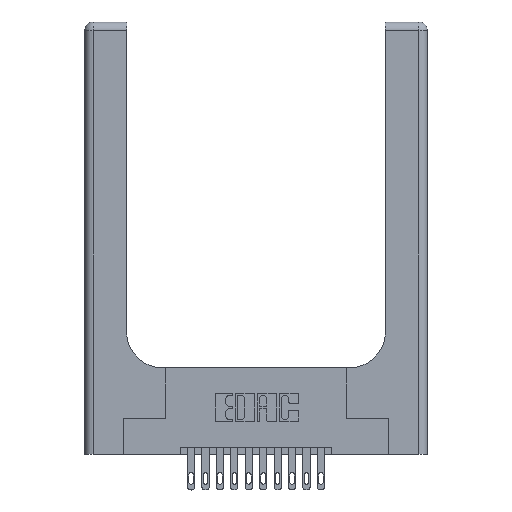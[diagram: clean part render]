
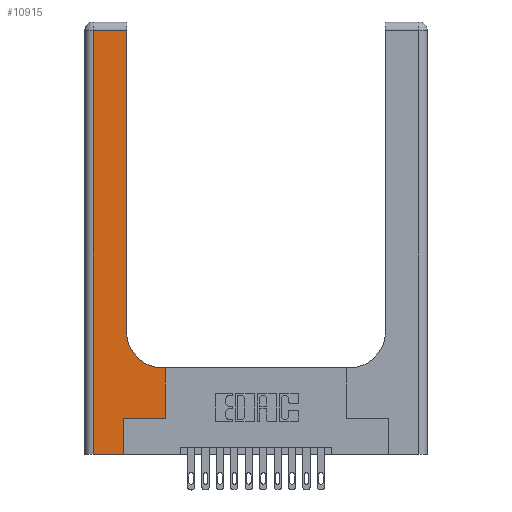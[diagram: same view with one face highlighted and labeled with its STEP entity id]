
A CAD part, top view. The second image highlights one B-rep face of the part: STEP entity #10915.
In plain terms, the highlighted planar face has unit normal (0, 0, 1).
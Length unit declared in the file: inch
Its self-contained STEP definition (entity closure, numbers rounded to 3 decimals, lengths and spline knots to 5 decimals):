
#44 = EDGE_CURVE ( 'NONE', #10128, #5933, #13331, .T. ) ;
#52 = VERTEX_POINT ( 'NONE', #16624 ) ;
#159 = EDGE_CURVE ( 'NONE', #2779, #11564, #11228, .T. ) ;
#255 = CARTESIAN_POINT ( 'NONE',  ( 0.269, 0., 0.37 ) ) ;
#813 = ORIENTED_EDGE ( 'NONE', *, *, #2667, .T. ) ;
#877 = VERTEX_POINT ( 'NONE', #5830 ) ;
#1017 = CARTESIAN_POINT ( 'NONE',  ( 0., 3., 0.37 ) ) ;
#1020 = ORIENTED_EDGE ( 'NONE', *, *, #2813, .T. ) ;
#1237 = CARTESIAN_POINT ( 'NONE',  ( 0.2915, 0.85, 0.37 ) ) ;
#1451 = CARTESIAN_POINT ( 'NONE',  ( 0.5415, 0.85, 0.37 ) ) ;
#1476 = FACE_OUTER_BOUND ( 'NONE', #13652, .T. ) ;
#1637 = EDGE_CURVE ( 'NONE', #7369, #5616, #4275, .T. ) ;
#1728 = VECTOR ( 'NONE', #9862, 39.37008 ) ;
#1870 = VECTOR ( 'NONE', #3087, 39.37008 ) ;
#2667 = EDGE_CURVE ( 'NONE', #7408, #52, #6954, .T. ) ;
#2746 = ORIENTED_EDGE ( 'NONE', *, *, #4909, .T. ) ;
#2756 = LINE ( 'NONE', #15110, #1728 ) ;
#2779 = VERTEX_POINT ( 'NONE', #5745 ) ;
#2813 = EDGE_CURVE ( 'NONE', #5616, #10128, #2756, .T. ) ;
#3087 = DIRECTION ( 'NONE',  ( 0., 1., 0. ) ) ;
#3137 = DIRECTION ( 'NONE',  ( -1., 0., 0. ) ) ;
#3143 = VECTOR ( 'NONE', #10471, 39.37008 ) ;
#3202 = CARTESIAN_POINT ( 'NONE',  ( 0.2915, 3., 0.37 ) ) ;
#3759 = EDGE_CURVE ( 'NONE', #52, #2779, #16509, .T. ) ;
#3787 = CARTESIAN_POINT ( 'NONE',  ( 0.269, 0.25, 0.37 ) ) ;
#3986 = LINE ( 'NONE', #3202, #11939 ) ;
#4275 = LINE ( 'NONE', #5670, #12419 ) ;
#4370 = DIRECTION ( 'NONE',  ( 0., 1., 0. ) ) ;
#4479 = CARTESIAN_POINT ( 'NONE',  ( 0.2915, 2.94, 0.37 ) ) ;
#4909 = EDGE_CURVE ( 'NONE', #5933, #877, #9811, .T. ) ;
#5306 = VECTOR ( 'NONE', #4370, 39.37008 ) ;
#5543 = CARTESIAN_POINT ( 'NONE',  ( 0.269, 0., 0.37 ) ) ;
#5598 = AXIS2_PLACEMENT_3D ( 'NONE', #1017, #15886, #15771 ) ;
#5616 = VERTEX_POINT ( 'NONE', #11672 ) ;
#5670 = CARTESIAN_POINT ( 'NONE',  ( 0., 2.94, 0.37 ) ) ;
#5745 = CARTESIAN_POINT ( 'NONE',  ( 0.5415, 0.6, 0.37 ) ) ;
#5830 = CARTESIAN_POINT ( 'NONE',  ( 0.269, 0.25, 0.37 ) ) ;
#5933 = VERTEX_POINT ( 'NONE', #5543 ) ;
#6586 = DIRECTION ( 'NONE',  ( 0., 0., -1. ) ) ;
#6954 = LINE ( 'NONE', #10886, #5306 ) ;
#7369 = VERTEX_POINT ( 'NONE', #4479 ) ;
#7408 = VERTEX_POINT ( 'NONE', #15059 ) ;
#7540 = ORIENTED_EDGE ( 'NONE', *, *, #10508, .T. ) ;
#7958 = CARTESIAN_POINT ( 'NONE',  ( 0.2915, 0.6, 0.37 ) ) ;
#8627 = ORIENTED_EDGE ( 'NONE', *, *, #159, .T. ) ;
#9721 = AXIS2_PLACEMENT_3D ( 'NONE', #1451, #6586, #9752 ) ;
#9752 = DIRECTION ( 'NONE',  ( 1., 0., 0. ) ) ;
#9811 = LINE ( 'NONE', #255, #1870 ) ;
#9862 = DIRECTION ( 'NONE',  ( 0., -1., 0. ) ) ;
#9909 = CARTESIAN_POINT ( 'NONE',  ( 0.06, 0., 0.37 ) ) ;
#9919 = DIRECTION ( 'NONE',  ( 1., 0., 0. ) ) ;
#10128 = VERTEX_POINT ( 'NONE', #9909 ) ;
#10471 = DIRECTION ( 'NONE',  ( -1., 0., 0. ) ) ;
#10508 = EDGE_CURVE ( 'NONE', #11564, #7369, #3986, .T. ) ;
#10886 = CARTESIAN_POINT ( 'NONE',  ( 0.5585, 0.25, 0.37 ) ) ;
#10915 = ADVANCED_FACE ( 'NONE', ( #1476 ), #16994, .F. ) ;
#11111 = CARTESIAN_POINT ( 'NONE',  ( 0., 0., 0.37 ) ) ;
#11203 = ORIENTED_EDGE ( 'NONE', *, *, #11535, .T. ) ;
#11228 = CIRCLE ( 'NONE', #9721, 0.25 ) ;
#11333 = ORIENTED_EDGE ( 'NONE', *, *, #3759, .T. ) ;
#11535 = EDGE_CURVE ( 'NONE', #877, #7408, #17094, .T. ) ;
#11564 = VERTEX_POINT ( 'NONE', #1237 ) ;
#11672 = CARTESIAN_POINT ( 'NONE',  ( 0.06, 2.94, 0.37 ) ) ;
#11939 = VECTOR ( 'NONE', #15438, 39.37008 ) ;
#12419 = VECTOR ( 'NONE', #3137, 39.37008 ) ;
#13331 = LINE ( 'NONE', #11111, #14360 ) ;
#13652 = EDGE_LOOP ( 'NONE', ( #7540, #16104, #1020, #15329, #2746, #11203, #813, #11333, #8627 ) ) ;
#13775 = VECTOR ( 'NONE', #14366, 39.37008 ) ;
#14360 = VECTOR ( 'NONE', #9919, 39.37008 ) ;
#14366 = DIRECTION ( 'NONE',  ( 1., 0., 0. ) ) ;
#15059 = CARTESIAN_POINT ( 'NONE',  ( 0.5585, 0.25, 0.37 ) ) ;
#15110 = CARTESIAN_POINT ( 'NONE',  ( 0.06, 3., 0.37 ) ) ;
#15329 = ORIENTED_EDGE ( 'NONE', *, *, #44, .T. ) ;
#15438 = DIRECTION ( 'NONE',  ( 0., 1., 0. ) ) ;
#15771 = DIRECTION ( 'NONE',  ( -1., 0., 0. ) ) ;
#15886 = DIRECTION ( 'NONE',  ( 0., 0., -1. ) ) ;
#16104 = ORIENTED_EDGE ( 'NONE', *, *, #1637, .T. ) ;
#16509 = LINE ( 'NONE', #7958, #3143 ) ;
#16624 = CARTESIAN_POINT ( 'NONE',  ( 0.5585, 0.6, 0.37 ) ) ;
#16994 = PLANE ( 'NONE',  #5598 ) ;
#17094 = LINE ( 'NONE', #3787, #13775 ) ;
